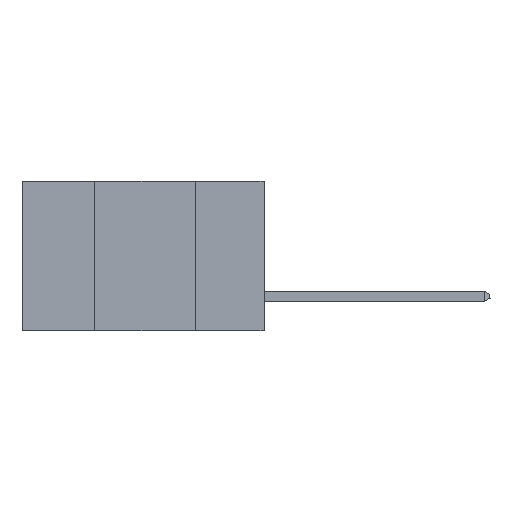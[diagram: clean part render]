
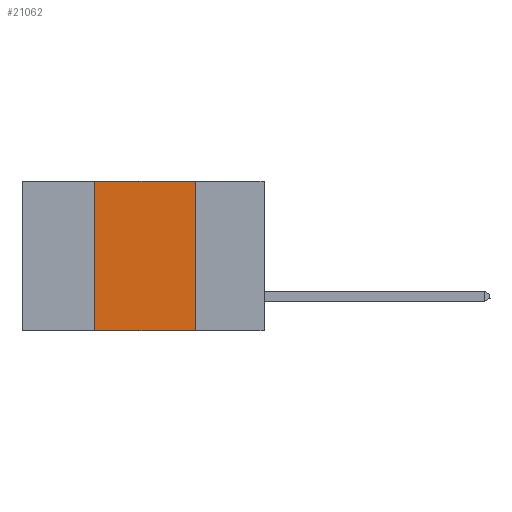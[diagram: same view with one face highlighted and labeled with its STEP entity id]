
A CAD part, left-side view. The second image highlights one B-rep face of the part: STEP entity #21062.
In plain terms, the highlighted planar face has unit normal (-1, 0, 0).
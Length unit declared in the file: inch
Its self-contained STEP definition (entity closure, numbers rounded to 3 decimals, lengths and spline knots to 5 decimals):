
#430 = ORIENTED_EDGE ( 'NONE', *, *, #12129, .F. ) ;
#3378 = DIRECTION ( 'NONE',  ( 1., 0., 0. ) ) ;
#3473 = DIRECTION ( 'NONE',  ( 0., 0., -1. ) ) ;
#3635 = ORIENTED_EDGE ( 'NONE', *, *, #23199, .F. ) ;
#3722 = VERTEX_POINT ( 'NONE', #26478 ) ;
#5004 = EDGE_CURVE ( 'NONE', #3722, #9672, #7624, .T. ) ;
#5076 = DIRECTION ( 'NONE',  ( 0., 0., -1. ) ) ;
#5842 = LINE ( 'NONE', #19301, #23262 ) ;
#5953 = CARTESIAN_POINT ( 'NONE',  ( 0., 0.42, 0. ) ) ;
#7328 = VERTEX_POINT ( 'NONE', #16563 ) ;
#7624 = LINE ( 'NONE', #17167, #23946 ) ;
#8144 = DIRECTION ( 'NONE',  ( 0., -1., 0. ) ) ;
#9672 = VERTEX_POINT ( 'NONE', #30732 ) ;
#10152 = DIRECTION ( 'NONE',  ( 0., 0., 1. ) ) ;
#12039 = LINE ( 'NONE', #17560, #20572 ) ;
#12129 = EDGE_CURVE ( 'NONE', #13727, #3722, #12039, .T. ) ;
#13112 = PLANE ( 'NONE',  #20546 ) ;
#13727 = VERTEX_POINT ( 'NONE', #5953 ) ;
#14279 = VECTOR ( 'NONE', #20058, 39.37008 ) ;
#16563 = CARTESIAN_POINT ( 'NONE',  ( 0., 0.42, -0.37 ) ) ;
#17167 = CARTESIAN_POINT ( 'NONE',  ( 0., 0.17, 0. ) ) ;
#17379 = ORIENTED_EDGE ( 'NONE', *, *, #27190, .T. ) ;
#17560 = CARTESIAN_POINT ( 'NONE',  ( 0., 0.6, 0. ) ) ;
#19301 = CARTESIAN_POINT ( 'NONE',  ( 0., 0.42, 0. ) ) ;
#19959 = CARTESIAN_POINT ( 'NONE',  ( 0., 0.6, -0.37 ) ) ;
#20058 = DIRECTION ( 'NONE',  ( 0., -1., 0. ) ) ;
#20546 = AXIS2_PLACEMENT_3D ( 'NONE', #22541, #3378, #3473 ) ;
#20572 = VECTOR ( 'NONE', #8144, 39.37008 ) ;
#21062 = ADVANCED_FACE ( 'NONE', ( #22283 ), #13112, .F. ) ;
#22283 = FACE_OUTER_BOUND ( 'NONE', #24385, .T. ) ;
#22541 = CARTESIAN_POINT ( 'NONE',  ( 0., 0.6, 0. ) ) ;
#23199 = EDGE_CURVE ( 'NONE', #7328, #13727, #5842, .T. ) ;
#23262 = VECTOR ( 'NONE', #10152, 39.37008 ) ;
#23946 = VECTOR ( 'NONE', #5076, 39.37008 ) ;
#24385 = EDGE_LOOP ( 'NONE', ( #26859, #430, #3635, #17379 ) ) ;
#25397 = LINE ( 'NONE', #19959, #14279 ) ;
#26478 = CARTESIAN_POINT ( 'NONE',  ( 0., 0.17, 0. ) ) ;
#26859 = ORIENTED_EDGE ( 'NONE', *, *, #5004, .F. ) ;
#27190 = EDGE_CURVE ( 'NONE', #7328, #9672, #25397, .T. ) ;
#30732 = CARTESIAN_POINT ( 'NONE',  ( 0., 0.17, -0.37 ) ) ;
